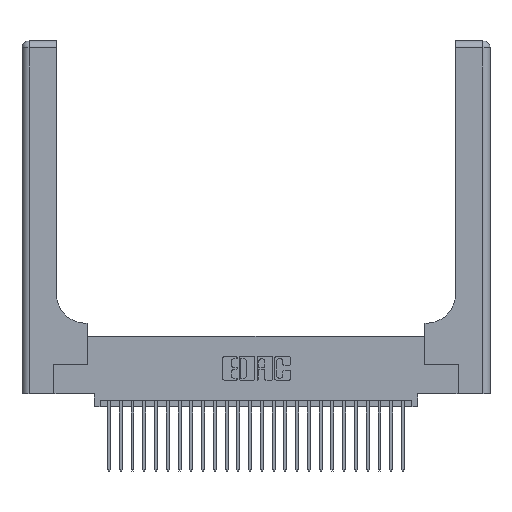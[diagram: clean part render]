
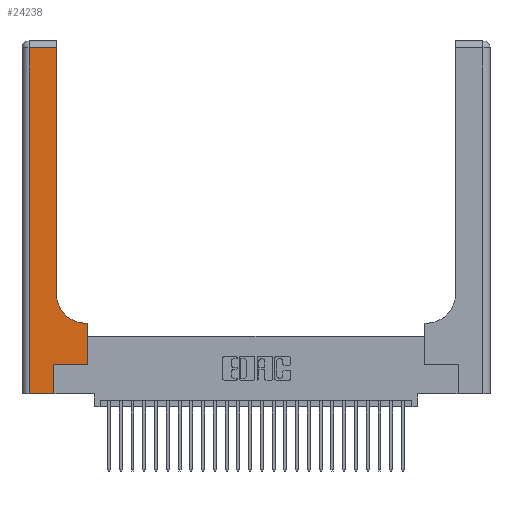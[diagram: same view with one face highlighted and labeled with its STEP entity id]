
A CAD part, top view. The second image highlights one B-rep face of the part: STEP entity #24238.
In plain terms, the highlighted planar face has unit normal (0, 0, 1).
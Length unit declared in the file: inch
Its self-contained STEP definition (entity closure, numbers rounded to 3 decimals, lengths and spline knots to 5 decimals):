
#241 = ORIENTED_EDGE ( 'NONE', *, *, #1812, .T. ) ;
#334 = VECTOR ( 'NONE', #13963, 39.37008 ) ;
#767 = DIRECTION ( 'NONE',  ( 0., 0., -1. ) ) ;
#1664 = CARTESIAN_POINT ( 'NONE',  ( 0.5585, 0.6, 0.37 ) ) ;
#1772 = DIRECTION ( 'NONE',  ( 1., 0., 0. ) ) ;
#1812 = EDGE_CURVE ( 'NONE', #18527, #21746, #19930, .T. ) ;
#1899 = CARTESIAN_POINT ( 'NONE',  ( 0., 3., 0.37 ) ) ;
#2510 = CARTESIAN_POINT ( 'NONE',  ( 0.5415, 0.6, 0.37 ) ) ;
#3463 = CARTESIAN_POINT ( 'NONE',  ( 0.06, 0., 0.37 ) ) ;
#4152 = EDGE_CURVE ( 'NONE', #26075, #27127, #6408, .T. ) ;
#4389 = CARTESIAN_POINT ( 'NONE',  ( 0.2915, 0.6, 0.37 ) ) ;
#4496 = VERTEX_POINT ( 'NONE', #20036 ) ;
#4959 = LINE ( 'NONE', #18893, #8704 ) ;
#5309 = CARTESIAN_POINT ( 'NONE',  ( 0.2915, 2.94, 0.37 ) ) ;
#5528 = LINE ( 'NONE', #11466, #23327 ) ;
#5906 = DIRECTION ( 'NONE',  ( 0., 0., -1. ) ) ;
#6408 = LINE ( 'NONE', #12772, #25535 ) ;
#7170 = CARTESIAN_POINT ( 'NONE',  ( 0.2915, 0.85, 0.37 ) ) ;
#7391 = CARTESIAN_POINT ( 'NONE',  ( 0.269, 0., 0.37 ) ) ;
#7754 = DIRECTION ( 'NONE',  ( 0., 1., 0. ) ) ;
#8101 = ORIENTED_EDGE ( 'NONE', *, *, #4152, .T. ) ;
#8704 = VECTOR ( 'NONE', #1772, 39.37008 ) ;
#9729 = ORIENTED_EDGE ( 'NONE', *, *, #14170, .T. ) ;
#10093 = ORIENTED_EDGE ( 'NONE', *, *, #13161, .T. ) ;
#10294 = CARTESIAN_POINT ( 'NONE',  ( 0.5585, 0.25, 0.37 ) ) ;
#10484 = ORIENTED_EDGE ( 'NONE', *, *, #25034, .T. ) ;
#11034 = CIRCLE ( 'NONE', #11961, 0.25 ) ;
#11398 = CARTESIAN_POINT ( 'NONE',  ( 0.5585, 0.25, 0.37 ) ) ;
#11416 = EDGE_CURVE ( 'NONE', #21746, #25285, #11034, .T. ) ;
#11466 = CARTESIAN_POINT ( 'NONE',  ( 0.2915, 3., 0.37 ) ) ;
#11833 = VERTEX_POINT ( 'NONE', #17605 ) ;
#11961 = AXIS2_PLACEMENT_3D ( 'NONE', #26641, #767, #20147 ) ;
#12281 = VECTOR ( 'NONE', #12359, 39.37008 ) ;
#12359 = DIRECTION ( 'NONE',  ( 1., 0., 0. ) ) ;
#12772 = CARTESIAN_POINT ( 'NONE',  ( 0., 2.94, 0.37 ) ) ;
#12861 = LINE ( 'NONE', #7391, #334 ) ;
#12870 = AXIS2_PLACEMENT_3D ( 'NONE', #1899, #5906, #27388 ) ;
#13161 = EDGE_CURVE ( 'NONE', #27674, #11833, #21961, .T. ) ;
#13238 = DIRECTION ( 'NONE',  ( -1., 0., 0. ) ) ;
#13834 = DIRECTION ( 'NONE',  ( 0., 1., 0. ) ) ;
#13854 = VECTOR ( 'NONE', #17138, 39.37008 ) ;
#13963 = DIRECTION ( 'NONE',  ( 0., 1., 0. ) ) ;
#14170 = EDGE_CURVE ( 'NONE', #11833, #4496, #12861, .T. ) ;
#14271 = PLANE ( 'NONE',  #12870 ) ;
#14605 = VECTOR ( 'NONE', #13238, 39.37008 ) ;
#15983 = ORIENTED_EDGE ( 'NONE', *, *, #23000, .T. ) ;
#16510 = VERTEX_POINT ( 'NONE', #10294 ) ;
#16987 = EDGE_LOOP ( 'NONE', ( #22153, #8101, #15983, #10093, #9729, #10484, #21445, #241, #21255 ) ) ;
#17138 = DIRECTION ( 'NONE',  ( 0., -1., 0. ) ) ;
#17605 = CARTESIAN_POINT ( 'NONE',  ( 0.269, 0., 0.37 ) ) ;
#18527 = VERTEX_POINT ( 'NONE', #1664 ) ;
#18662 = DIRECTION ( 'NONE',  ( -1., 0., 0. ) ) ;
#18893 = CARTESIAN_POINT ( 'NONE',  ( 0.269, 0.25, 0.37 ) ) ;
#19183 = LINE ( 'NONE', #11398, #23545 ) ;
#19930 = LINE ( 'NONE', #4389, #14605 ) ;
#20036 = CARTESIAN_POINT ( 'NONE',  ( 0.269, 0.25, 0.37 ) ) ;
#20105 = FACE_OUTER_BOUND ( 'NONE', #16987, .T. ) ;
#20147 = DIRECTION ( 'NONE',  ( 1., 0., 0. ) ) ;
#20881 = CARTESIAN_POINT ( 'NONE',  ( 0.06, 2.94, 0.37 ) ) ;
#21255 = ORIENTED_EDGE ( 'NONE', *, *, #11416, .T. ) ;
#21445 = ORIENTED_EDGE ( 'NONE', *, *, #23343, .T. ) ;
#21746 = VERTEX_POINT ( 'NONE', #2510 ) ;
#21961 = LINE ( 'NONE', #26973, #12281 ) ;
#22153 = ORIENTED_EDGE ( 'NONE', *, *, #27602, .T. ) ;
#23000 = EDGE_CURVE ( 'NONE', #27127, #27674, #25908, .T. ) ;
#23327 = VECTOR ( 'NONE', #13834, 39.37008 ) ;
#23343 = EDGE_CURVE ( 'NONE', #16510, #18527, #19183, .T. ) ;
#23513 = CARTESIAN_POINT ( 'NONE',  ( 0.06, 3., 0.37 ) ) ;
#23545 = VECTOR ( 'NONE', #7754, 39.37008 ) ;
#24238 = ADVANCED_FACE ( 'NONE', ( #20105 ), #14271, .F. ) ;
#25034 = EDGE_CURVE ( 'NONE', #4496, #16510, #4959, .T. ) ;
#25285 = VERTEX_POINT ( 'NONE', #7170 ) ;
#25535 = VECTOR ( 'NONE', #18662, 39.37008 ) ;
#25908 = LINE ( 'NONE', #23513, #13854 ) ;
#26075 = VERTEX_POINT ( 'NONE', #5309 ) ;
#26641 = CARTESIAN_POINT ( 'NONE',  ( 0.5415, 0.85, 0.37 ) ) ;
#26973 = CARTESIAN_POINT ( 'NONE',  ( 0., 0., 0.37 ) ) ;
#27127 = VERTEX_POINT ( 'NONE', #20881 ) ;
#27388 = DIRECTION ( 'NONE',  ( -1., 0., 0. ) ) ;
#27602 = EDGE_CURVE ( 'NONE', #25285, #26075, #5528, .T. ) ;
#27674 = VERTEX_POINT ( 'NONE', #3463 ) ;
